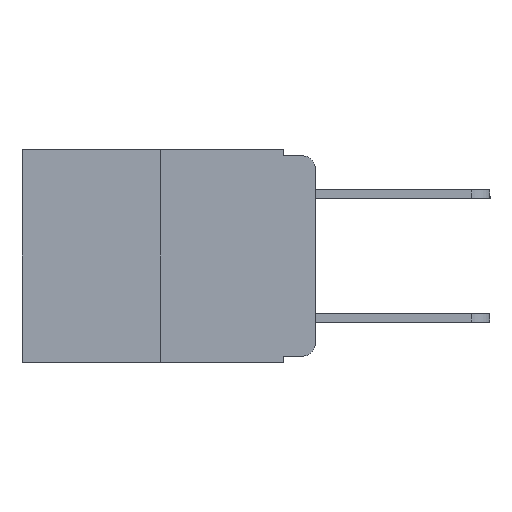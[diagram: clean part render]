
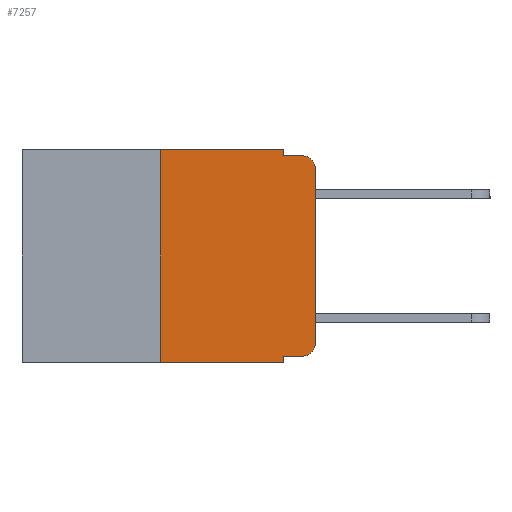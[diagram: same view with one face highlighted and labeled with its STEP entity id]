
A CAD part, left-side view. The second image highlights one B-rep face of the part: STEP entity #7257.
In plain terms, the highlighted planar face has unit normal (-1, 0, 0).
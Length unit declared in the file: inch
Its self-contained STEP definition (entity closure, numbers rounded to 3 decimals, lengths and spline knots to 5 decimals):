
#182 = DIRECTION ( 'NONE',  ( 0., 0., -1. ) ) ;
#242 = FACE_OUTER_BOUND ( 'NONE', #7572, .T. ) ;
#480 = CARTESIAN_POINT ( 'NONE',  ( 0., 0.051, -0.01 ) ) ;
#509 = VERTEX_POINT ( 'NONE', #10825 ) ;
#788 = VECTOR ( 'NONE', #5184, 39.37008 ) ;
#791 = EDGE_CURVE ( 'NONE', #4386, #4251, #1946, .T. ) ;
#792 = DIRECTION ( 'NONE',  ( -1., 0., 0. ) ) ;
#844 = VECTOR ( 'NONE', #3019, 39.37008 ) ;
#896 = DIRECTION ( 'NONE',  ( 0., 0., -1. ) ) ;
#1081 = CARTESIAN_POINT ( 'NONE',  ( 0., 0.473, -0.343 ) ) ;
#1358 = VERTEX_POINT ( 'NONE', #10521 ) ;
#1407 = ORIENTED_EDGE ( 'NONE', *, *, #8812, .T. ) ;
#1510 = CARTESIAN_POINT ( 'NONE',  ( 0., 0.02, -0.01 ) ) ;
#1788 = EDGE_CURVE ( 'NONE', #4386, #509, #9728, .T. ) ;
#1946 = LINE ( 'NONE', #4376, #4934 ) ;
#1956 = ORIENTED_EDGE ( 'NONE', *, *, #7512, .F. ) ;
#2240 = ORIENTED_EDGE ( 'NONE', *, *, #6116, .T. ) ;
#2460 = LINE ( 'NONE', #8498, #6827 ) ;
#2549 = LINE ( 'NONE', #5945, #7192 ) ;
#2745 = CARTESIAN_POINT ( 'NONE',  ( 0., 0.051, 0. ) ) ;
#2818 = EDGE_CURVE ( 'NONE', #4745, #8318, #4095, .T. ) ;
#2920 = CARTESIAN_POINT ( 'NONE',  ( 0., 0.25, -0.343 ) ) ;
#2954 = CARTESIAN_POINT ( 'NONE',  ( 0., 0.051, -0.343 ) ) ;
#3019 = DIRECTION ( 'NONE',  ( 0., -1., 0. ) ) ;
#3412 = CIRCLE ( 'NONE', #9602, 0.02 ) ;
#3414 = LINE ( 'NONE', #1081, #8469 ) ;
#3625 = PLANE ( 'NONE',  #10736 ) ;
#4095 = LINE ( 'NONE', #2745, #788 ) ;
#4251 = VERTEX_POINT ( 'NONE', #2954 ) ;
#4376 = CARTESIAN_POINT ( 'NONE',  ( 0., 0.051, 0. ) ) ;
#4386 = VERTEX_POINT ( 'NONE', #10893 ) ;
#4709 = LINE ( 'NONE', #6371, #5432 ) ;
#4745 = VERTEX_POINT ( 'NONE', #6381 ) ;
#4934 = VECTOR ( 'NONE', #182, 39.37008 ) ;
#5159 = ORIENTED_EDGE ( 'NONE', *, *, #7085, .F. ) ;
#5184 = DIRECTION ( 'NONE',  ( 0., 0., -1. ) ) ;
#5289 = AXIS2_PLACEMENT_3D ( 'NONE', #7649, #792, #896 ) ;
#5432 = VECTOR ( 'NONE', #10703, 39.37008 ) ;
#5518 = CARTESIAN_POINT ( 'NONE',  ( 0., 0.051, -0.333 ) ) ;
#5578 = ORIENTED_EDGE ( 'NONE', *, *, #1788, .T. ) ;
#5752 = ORIENTED_EDGE ( 'NONE', *, *, #8494, .T. ) ;
#5945 = CARTESIAN_POINT ( 'NONE',  ( 0., 0.473, 0. ) ) ;
#6116 = EDGE_CURVE ( 'NONE', #509, #1358, #3412, .T. ) ;
#6371 = CARTESIAN_POINT ( 'NONE',  ( 0., 0., 0. ) ) ;
#6381 = CARTESIAN_POINT ( 'NONE',  ( 0., 0.051, 0. ) ) ;
#6382 = ORIENTED_EDGE ( 'NONE', *, *, #7791, .T. ) ;
#6452 = CARTESIAN_POINT ( 'NONE',  ( 0., 0.25, 0. ) ) ;
#6605 = ORIENTED_EDGE ( 'NONE', *, *, #791, .F. ) ;
#6765 = DIRECTION ( 'NONE',  ( 0., -1., 0. ) ) ;
#6779 = DIRECTION ( 'NONE',  ( 0., -1., 0. ) ) ;
#6827 = VECTOR ( 'NONE', #6779, 39.37008 ) ;
#7004 = DIRECTION ( 'NONE',  ( 1., 0., 0. ) ) ;
#7066 = ORIENTED_EDGE ( 'NONE', *, *, #2818, .F. ) ;
#7085 = EDGE_CURVE ( 'NONE', #8318, #7343, #2460, .T. ) ;
#7192 = VECTOR ( 'NONE', #6765, 39.37008 ) ;
#7257 = ADVANCED_FACE ( 'NONE', ( #242 ), #3625, .F. ) ;
#7343 = VERTEX_POINT ( 'NONE', #1510 ) ;
#7425 = LINE ( 'NONE', #10809, #7879 ) ;
#7512 = EDGE_CURVE ( 'NONE', #10388, #4745, #2549, .T. ) ;
#7572 = EDGE_LOOP ( 'NONE', ( #6382, #1407, #5159, #7066, #1956, #8900, #5752, #6605, #5578, #2240 ) ) ;
#7591 = VERTEX_POINT ( 'NONE', #8816 ) ;
#7649 = CARTESIAN_POINT ( 'NONE',  ( 0., 0.02, -0.03 ) ) ;
#7791 = EDGE_CURVE ( 'NONE', #1358, #7591, #4709, .T. ) ;
#7879 = VECTOR ( 'NONE', #8632, 39.37008 ) ;
#8057 = EDGE_CURVE ( 'NONE', #9561, #10388, #7425, .T. ) ;
#8318 = VERTEX_POINT ( 'NONE', #480 ) ;
#8469 = VECTOR ( 'NONE', #10227, 39.37008 ) ;
#8494 = EDGE_CURVE ( 'NONE', #9561, #4251, #3414, .T. ) ;
#8498 = CARTESIAN_POINT ( 'NONE',  ( 0., 0.051, -0.01 ) ) ;
#8529 = CARTESIAN_POINT ( 'NONE',  ( 0., 0.02, -0.313 ) ) ;
#8608 = DIRECTION ( 'NONE',  ( 0., 0., -1. ) ) ;
#8632 = DIRECTION ( 'NONE',  ( 0., 0., 1. ) ) ;
#8781 = CARTESIAN_POINT ( 'NONE',  ( 0., 0.473, 0. ) ) ;
#8812 = EDGE_CURVE ( 'NONE', #7591, #7343, #10789, .T. ) ;
#8816 = CARTESIAN_POINT ( 'NONE',  ( 0., 0., -0.03 ) ) ;
#8900 = ORIENTED_EDGE ( 'NONE', *, *, #8057, .F. ) ;
#9321 = DIRECTION ( 'NONE',  ( 0., 0., -1. ) ) ;
#9561 = VERTEX_POINT ( 'NONE', #2920 ) ;
#9602 = AXIS2_PLACEMENT_3D ( 'NONE', #8529, #10667, #9321 ) ;
#9728 = LINE ( 'NONE', #5518, #844 ) ;
#10227 = DIRECTION ( 'NONE',  ( 0., -1., 0. ) ) ;
#10388 = VERTEX_POINT ( 'NONE', #6452 ) ;
#10521 = CARTESIAN_POINT ( 'NONE',  ( 0., 0., -0.313 ) ) ;
#10667 = DIRECTION ( 'NONE',  ( -1., 0., 0. ) ) ;
#10703 = DIRECTION ( 'NONE',  ( 0., 0., 1. ) ) ;
#10736 = AXIS2_PLACEMENT_3D ( 'NONE', #8781, #7004, #8608 ) ;
#10789 = CIRCLE ( 'NONE', #5289, 0.02 ) ;
#10809 = CARTESIAN_POINT ( 'NONE',  ( 0., 0.25, 0. ) ) ;
#10825 = CARTESIAN_POINT ( 'NONE',  ( 0., 0.02, -0.333 ) ) ;
#10893 = CARTESIAN_POINT ( 'NONE',  ( 0., 0.051, -0.333 ) ) ;
